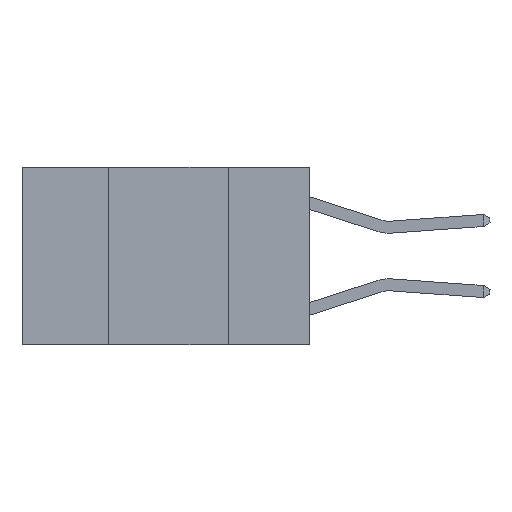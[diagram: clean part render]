
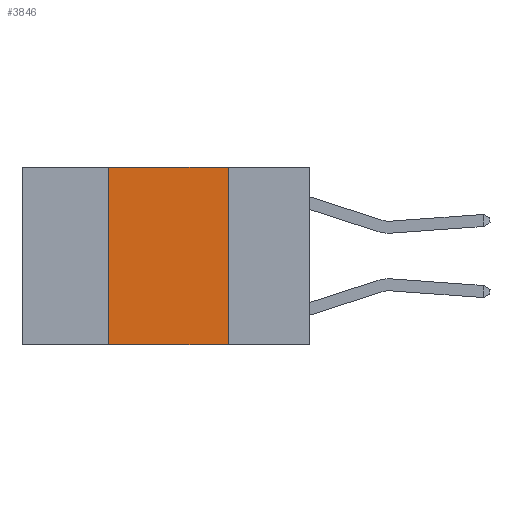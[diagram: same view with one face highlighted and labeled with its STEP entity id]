
A CAD part, left-side view. The second image highlights one B-rep face of the part: STEP entity #3846.
In plain terms, the highlighted planar face has unit normal (-1, 0, 0).
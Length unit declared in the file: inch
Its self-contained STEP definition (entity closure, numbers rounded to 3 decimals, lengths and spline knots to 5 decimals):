
#38 = CARTESIAN_POINT ( 'NONE',  ( 0., 0.6, 0. ) ) ;
#149 = DIRECTION ( 'NONE',  ( 0., 0., 1. ) ) ;
#241 = ORIENTED_EDGE ( 'NONE', *, *, #3804, .F. ) ;
#316 = ORIENTED_EDGE ( 'NONE', *, *, #3484, .F. ) ;
#1612 = DIRECTION ( 'NONE',  ( 1., 0., 0. ) ) ;
#1702 = VERTEX_POINT ( 'NONE', #2778 ) ;
#1717 = DIRECTION ( 'NONE',  ( 0., -1., 0. ) ) ;
#1841 = CARTESIAN_POINT ( 'NONE',  ( 0., 0.17, -0.37 ) ) ;
#2118 = PLANE ( 'NONE',  #7926 ) ;
#2162 = CARTESIAN_POINT ( 'NONE',  ( 0., 0.6, 0. ) ) ;
#2241 = ORIENTED_EDGE ( 'NONE', *, *, #7355, .F. ) ;
#2778 = CARTESIAN_POINT ( 'NONE',  ( 0., 0.42, -0.37 ) ) ;
#3145 = LINE ( 'NONE', #2162, #8235 ) ;
#3254 = VECTOR ( 'NONE', #7811, 39.37008 ) ;
#3435 = CARTESIAN_POINT ( 'NONE',  ( 0., 0.17, 0. ) ) ;
#3484 = EDGE_CURVE ( 'NONE', #3701, #5786, #3145, .T. ) ;
#3669 = DIRECTION ( 'NONE',  ( 0., 0., -1. ) ) ;
#3694 = ORIENTED_EDGE ( 'NONE', *, *, #6701, .T. ) ;
#3701 = VERTEX_POINT ( 'NONE', #5357 ) ;
#3765 = FACE_OUTER_BOUND ( 'NONE', #6280, .T. ) ;
#3804 = EDGE_CURVE ( 'NONE', #5786, #4286, #6103, .T. ) ;
#3846 = ADVANCED_FACE ( 'NONE', ( #3765 ), #2118, .F. ) ;
#3899 = DIRECTION ( 'NONE',  ( 0., 0., -1. ) ) ;
#4286 = VERTEX_POINT ( 'NONE', #1841 ) ;
#4625 = CARTESIAN_POINT ( 'NONE',  ( 0., 0.17, 0. ) ) ;
#5357 = CARTESIAN_POINT ( 'NONE',  ( 0., 0.42, 0. ) ) ;
#5680 = VECTOR ( 'NONE', #3899, 39.37008 ) ;
#5738 = CARTESIAN_POINT ( 'NONE',  ( 0., 0.6, -0.37 ) ) ;
#5786 = VERTEX_POINT ( 'NONE', #3435 ) ;
#6103 = LINE ( 'NONE', #4625, #5680 ) ;
#6191 = VECTOR ( 'NONE', #149, 39.37008 ) ;
#6280 = EDGE_LOOP ( 'NONE', ( #241, #316, #2241, #3694 ) ) ;
#6701 = EDGE_CURVE ( 'NONE', #1702, #4286, #8745, .T. ) ;
#6993 = CARTESIAN_POINT ( 'NONE',  ( 0., 0.42, 0. ) ) ;
#7355 = EDGE_CURVE ( 'NONE', #1702, #3701, #8025, .T. ) ;
#7811 = DIRECTION ( 'NONE',  ( 0., -1., 0. ) ) ;
#7926 = AXIS2_PLACEMENT_3D ( 'NONE', #38, #1612, #3669 ) ;
#8025 = LINE ( 'NONE', #6993, #6191 ) ;
#8235 = VECTOR ( 'NONE', #1717, 39.37008 ) ;
#8745 = LINE ( 'NONE', #5738, #3254 ) ;
